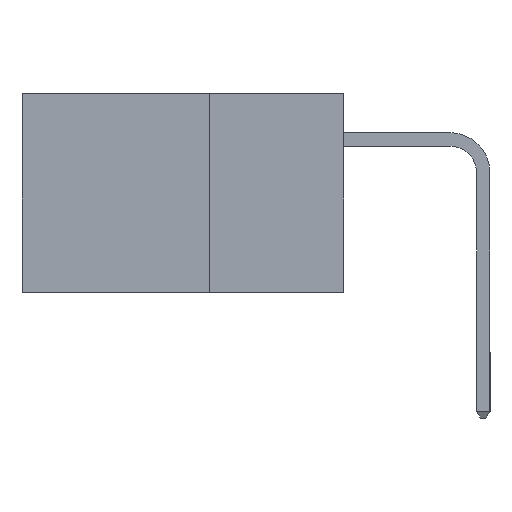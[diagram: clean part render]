
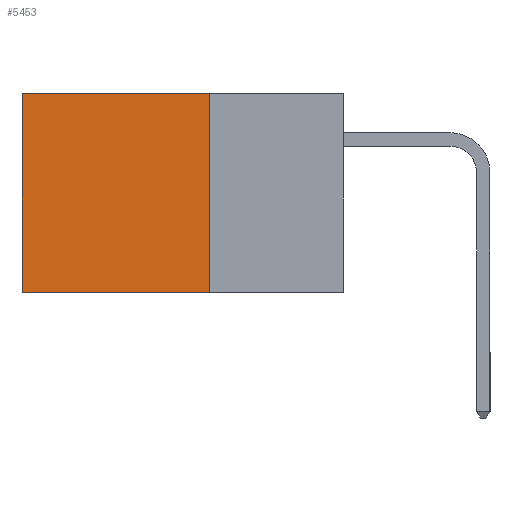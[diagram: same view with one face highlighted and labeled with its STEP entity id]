
A CAD part, left-side view. The second image highlights one B-rep face of the part: STEP entity #5453.
In plain terms, the highlighted planar face has unit normal (-1, 0, 0).
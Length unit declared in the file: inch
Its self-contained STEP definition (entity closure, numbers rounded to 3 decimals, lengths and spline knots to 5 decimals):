
#6 = ORIENTED_EDGE ( 'NONE', *, *, #279, .F. ) ;
#157 = DIRECTION ( 'NONE',  ( 0., 0., -1. ) ) ;
#279 = EDGE_CURVE ( 'NONE', #8311, #7601, #12620, .T. ) ;
#713 = PLANE ( 'NONE',  #13064 ) ;
#841 = VECTOR ( 'NONE', #8727, 39.37008 ) ;
#1311 = VECTOR ( 'NONE', #157, 39.37008 ) ;
#1891 = VECTOR ( 'NONE', #6252, 39.37008 ) ;
#1928 = LINE ( 'NONE', #6218, #10806 ) ;
#2273 = CARTESIAN_POINT ( 'NONE',  ( 0.2615, 0.25, -0.37 ) ) ;
#2698 = EDGE_CURVE ( 'NONE', #7601, #9770, #11929, .T. ) ;
#2766 = CARTESIAN_POINT ( 'NONE',  ( 0.2615, 0.25, -0.37 ) ) ;
#5109 = CARTESIAN_POINT ( 'NONE',  ( 0.2615, 0.25, -0.37 ) ) ;
#5174 = EDGE_CURVE ( 'NONE', #13858, #9770, #6643, .T. ) ;
#5453 = ADVANCED_FACE ( 'NONE', ( #5999 ), #713, .F. ) ;
#5989 = ORIENTED_EDGE ( 'NONE', *, *, #5174, .T. ) ;
#5999 = FACE_OUTER_BOUND ( 'NONE', #8768, .T. ) ;
#6117 = CARTESIAN_POINT ( 'NONE',  ( 0.2615, 0.25, -0.37 ) ) ;
#6218 = CARTESIAN_POINT ( 'NONE',  ( 0.2615, 0.25, 0. ) ) ;
#6220 = CARTESIAN_POINT ( 'NONE',  ( 0.2615, 0.6, -0.37 ) ) ;
#6252 = DIRECTION ( 'NONE',  ( 0., 0., -1. ) ) ;
#6643 = LINE ( 'NONE', #9811, #1311 ) ;
#7329 = DIRECTION ( 'NONE',  ( 1., 0., 0. ) ) ;
#7601 = VERTEX_POINT ( 'NONE', #6117 ) ;
#8013 = ORIENTED_EDGE ( 'NONE', *, *, #2698, .F. ) ;
#8311 = VERTEX_POINT ( 'NONE', #11742 ) ;
#8727 = DIRECTION ( 'NONE',  ( 0., 1., 0. ) ) ;
#8768 = EDGE_LOOP ( 'NONE', ( #5989, #8013, #6, #10224 ) ) ;
#9770 = VERTEX_POINT ( 'NONE', #6220 ) ;
#9811 = CARTESIAN_POINT ( 'NONE',  ( 0.2615, 0.6, -0.37 ) ) ;
#10224 = ORIENTED_EDGE ( 'NONE', *, *, #13775, .T. ) ;
#10496 = DIRECTION ( 'NONE',  ( 0., 1., 0. ) ) ;
#10806 = VECTOR ( 'NONE', #10496, 39.37008 ) ;
#10864 = CARTESIAN_POINT ( 'NONE',  ( 0.2615, 0.6, 0. ) ) ;
#11649 = DIRECTION ( 'NONE',  ( 0., 0., -1. ) ) ;
#11742 = CARTESIAN_POINT ( 'NONE',  ( 0.2615, 0.25, 0. ) ) ;
#11929 = LINE ( 'NONE', #2273, #841 ) ;
#12620 = LINE ( 'NONE', #5109, #1891 ) ;
#13064 = AXIS2_PLACEMENT_3D ( 'NONE', #2766, #7329, #11649 ) ;
#13775 = EDGE_CURVE ( 'NONE', #8311, #13858, #1928, .T. ) ;
#13858 = VERTEX_POINT ( 'NONE', #10864 ) ;
